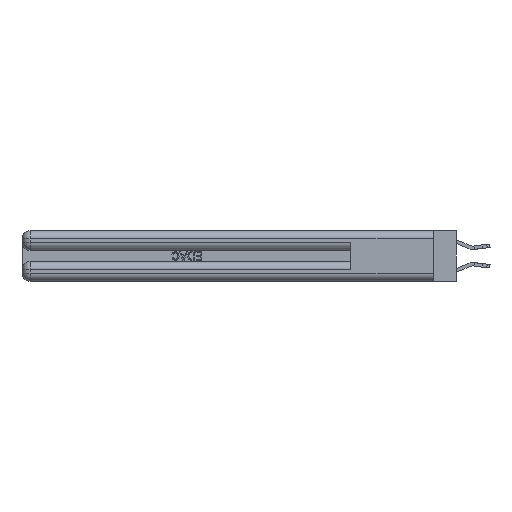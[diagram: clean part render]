
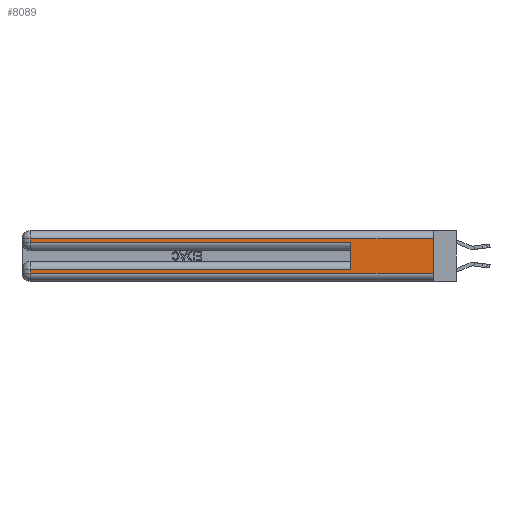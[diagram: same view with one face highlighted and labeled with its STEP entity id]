
A CAD part, left-side view. The second image highlights one B-rep face of the part: STEP entity #8089.
In plain terms, the highlighted planar face has unit normal (-1, 0, 0).
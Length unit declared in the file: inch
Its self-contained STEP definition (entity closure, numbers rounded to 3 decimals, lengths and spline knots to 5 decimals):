
#270 = VECTOR ( 'NONE', #28000, 39.37008 ) ;
#637 = CARTESIAN_POINT ( 'NONE',  ( 0., 0., 0.31 ) ) ;
#847 = ORIENTED_EDGE ( 'NONE', *, *, #26283, .F. ) ;
#1205 = VERTEX_POINT ( 'NONE', #12228 ) ;
#1470 = DIRECTION ( 'NONE',  ( 1., 0., 0. ) ) ;
#1594 = VECTOR ( 'NONE', #8580, 39.37008 ) ;
#1702 = DIRECTION ( 'NONE',  ( 0., 0., -1. ) ) ;
#2252 = ORIENTED_EDGE ( 'NONE', *, *, #2826, .T. ) ;
#2395 = VERTEX_POINT ( 'NONE', #3380 ) ;
#2691 = LINE ( 'NONE', #20160, #10906 ) ;
#2826 = EDGE_CURVE ( 'NONE', #2395, #10548, #18510, .T. ) ;
#3380 = CARTESIAN_POINT ( 'NONE',  ( 0., 2.94, 0.085 ) ) ;
#4336 = VECTOR ( 'NONE', #20358, 39.37008 ) ;
#4816 = ORIENTED_EDGE ( 'NONE', *, *, #15465, .T. ) ;
#4891 = ORIENTED_EDGE ( 'NONE', *, *, #13300, .T. ) ;
#5456 = LINE ( 'NONE', #22928, #4336 ) ;
#6706 = CARTESIAN_POINT ( 'NONE',  ( 0., 0., 0.37 ) ) ;
#6973 = AXIS2_PLACEMENT_3D ( 'NONE', #10808, #1470, #14523 ) ;
#7045 = ORIENTED_EDGE ( 'NONE', *, *, #9229, .F. ) ;
#7077 = EDGE_CURVE ( 'NONE', #10941, #19848, #5456, .T. ) ;
#7207 = CARTESIAN_POINT ( 'NONE',  ( 0., 2.94, 0.31 ) ) ;
#8050 = DIRECTION ( 'NONE',  ( 0., 0., -1. ) ) ;
#8089 = ADVANCED_FACE ( 'NONE', ( #21104 ), #25970, .F. ) ;
#8580 = DIRECTION ( 'NONE',  ( 0., 1., 0. ) ) ;
#8840 = DIRECTION ( 'NONE',  ( 0., 0., 1. ) ) ;
#9127 = VECTOR ( 'NONE', #1702, 39.37008 ) ;
#9229 = EDGE_CURVE ( 'NONE', #14651, #1205, #21889, .T. ) ;
#10548 = VERTEX_POINT ( 'NONE', #26595 ) ;
#10727 = DIRECTION ( 'NONE',  ( 0., 0., -1. ) ) ;
#10808 = CARTESIAN_POINT ( 'NONE',  ( 0., 0., 0.37 ) ) ;
#10906 = VECTOR ( 'NONE', #8840, 39.37008 ) ;
#10941 = VERTEX_POINT ( 'NONE', #21834 ) ;
#12228 = CARTESIAN_POINT ( 'NONE',  ( 0., 0., 0.06 ) ) ;
#12519 = VERTEX_POINT ( 'NONE', #7207 ) ;
#12880 = LINE ( 'NONE', #22190, #1594 ) ;
#13300 = EDGE_CURVE ( 'NONE', #25336, #2395, #12880, .T. ) ;
#13509 = VECTOR ( 'NONE', #8050, 39.37008 ) ;
#14476 = CARTESIAN_POINT ( 'NONE',  ( 0., 2.94, 0.37 ) ) ;
#14523 = DIRECTION ( 'NONE',  ( 0., 0., -1. ) ) ;
#14651 = VERTEX_POINT ( 'NONE', #24519 ) ;
#15465 = EDGE_CURVE ( 'NONE', #14651, #12519, #24449, .T. ) ;
#15903 = CARTESIAN_POINT ( 'NONE',  ( 0., 0.6, 0.085 ) ) ;
#16537 = CARTESIAN_POINT ( 'NONE',  ( 0., 2.94, 0.37 ) ) ;
#17039 = EDGE_CURVE ( 'NONE', #10548, #1205, #21429, .T. ) ;
#18274 = ORIENTED_EDGE ( 'NONE', *, *, #24953, .T. ) ;
#18510 = LINE ( 'NONE', #16537, #13509 ) ;
#19291 = CARTESIAN_POINT ( 'NONE',  ( 0., 0., 0.06 ) ) ;
#19848 = VERTEX_POINT ( 'NONE', #24421 ) ;
#20160 = CARTESIAN_POINT ( 'NONE',  ( 0., 0.6, 0.145 ) ) ;
#20358 = DIRECTION ( 'NONE',  ( 0., -1., 0. ) ) ;
#21104 = FACE_OUTER_BOUND ( 'NONE', #26871, .T. ) ;
#21334 = LINE ( 'NONE', #14476, #9127 ) ;
#21429 = LINE ( 'NONE', #19291, #270 ) ;
#21834 = CARTESIAN_POINT ( 'NONE',  ( 0., 2.94, 0.285 ) ) ;
#21889 = LINE ( 'NONE', #6706, #23121 ) ;
#22165 = DIRECTION ( 'NONE',  ( 0., 1., 0. ) ) ;
#22190 = CARTESIAN_POINT ( 'NONE',  ( 0., 0., 0.085 ) ) ;
#22928 = CARTESIAN_POINT ( 'NONE',  ( 0., 0., 0.285 ) ) ;
#23121 = VECTOR ( 'NONE', #10727, 39.37008 ) ;
#23368 = ORIENTED_EDGE ( 'NONE', *, *, #17039, .T. ) ;
#24303 = ORIENTED_EDGE ( 'NONE', *, *, #7077, .T. ) ;
#24421 = CARTESIAN_POINT ( 'NONE',  ( 0., 0.6, 0.285 ) ) ;
#24449 = LINE ( 'NONE', #637, #24624 ) ;
#24519 = CARTESIAN_POINT ( 'NONE',  ( 0., 0., 0.31 ) ) ;
#24624 = VECTOR ( 'NONE', #22165, 39.37008 ) ;
#24953 = EDGE_CURVE ( 'NONE', #12519, #10941, #21334, .T. ) ;
#25336 = VERTEX_POINT ( 'NONE', #15903 ) ;
#25970 = PLANE ( 'NONE',  #6973 ) ;
#26283 = EDGE_CURVE ( 'NONE', #25336, #19848, #2691, .T. ) ;
#26595 = CARTESIAN_POINT ( 'NONE',  ( 0., 2.94, 0.06 ) ) ;
#26871 = EDGE_LOOP ( 'NONE', ( #7045, #4816, #18274, #24303, #847, #4891, #2252, #23368 ) ) ;
#28000 = DIRECTION ( 'NONE',  ( 0., -1., 0. ) ) ;
